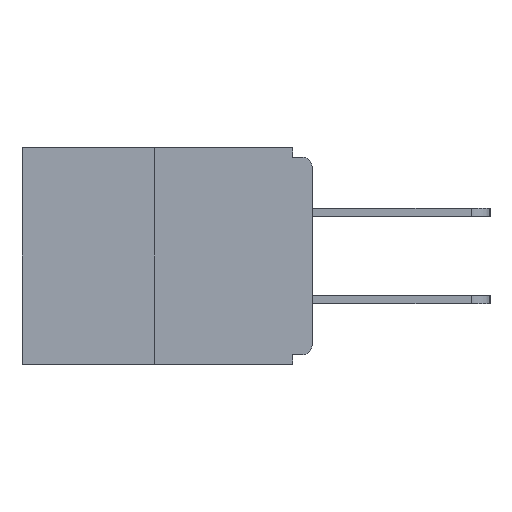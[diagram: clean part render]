
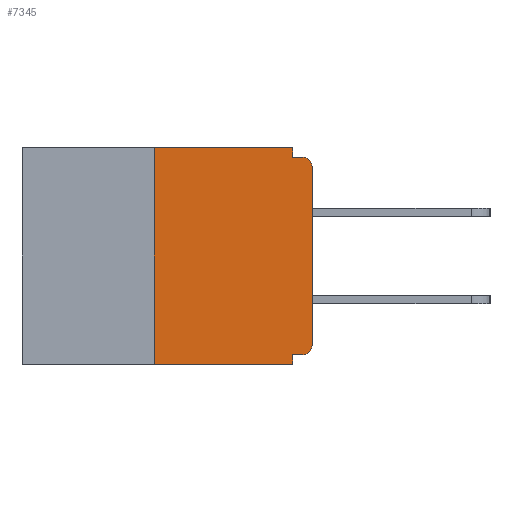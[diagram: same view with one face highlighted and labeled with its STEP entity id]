
A CAD part, left-side view. The second image highlights one B-rep face of the part: STEP entity #7345.
In plain terms, the highlighted planar face has unit normal (-1, 0, 0).
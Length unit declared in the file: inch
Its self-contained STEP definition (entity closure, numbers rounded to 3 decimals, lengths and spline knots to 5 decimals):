
#115 = CARTESIAN_POINT ( 'NONE',  ( 0., 0.015, -0.313 ) ) ;
#485 = EDGE_CURVE ( 'NONE', #3278, #4125, #10283, .T. ) ;
#529 = LINE ( 'NONE', #5410, #9290 ) ;
#544 = CARTESIAN_POINT ( 'NONE',  ( 0., 0.031, -0.328 ) ) ;
#545 = ORIENTED_EDGE ( 'NONE', *, *, #9384, .T. ) ;
#807 = ORIENTED_EDGE ( 'NONE', *, *, #485, .T. ) ;
#889 = EDGE_CURVE ( 'NONE', #6233, #6320, #529, .T. ) ;
#1041 = DIRECTION ( 'NONE',  ( -1., 0., 0. ) ) ;
#1102 = EDGE_CURVE ( 'NONE', #6320, #8349, #2236, .T. ) ;
#1229 = CARTESIAN_POINT ( 'NONE',  ( 0., 0.25, 0. ) ) ;
#1244 = EDGE_CURVE ( 'NONE', #6233, #3278, #9673, .T. ) ;
#1288 = CARTESIAN_POINT ( 'NONE',  ( 0., 0.015, -0.03 ) ) ;
#1404 = VERTEX_POINT ( 'NONE', #2201 ) ;
#1452 = VECTOR ( 'NONE', #3932, 39.37008 ) ;
#2037 = LINE ( 'NONE', #1229, #6083 ) ;
#2065 = VERTEX_POINT ( 'NONE', #5944 ) ;
#2121 = EDGE_LOOP ( 'NONE', ( #9521, #6067, #545, #6357, #8438, #2756, #807, #8352, #10331, #3234 ) ) ;
#2174 = CARTESIAN_POINT ( 'NONE',  ( 0., 0.031, -0.343 ) ) ;
#2178 = VECTOR ( 'NONE', #4045, 39.37008 ) ;
#2180 = LINE ( 'NONE', #8545, #1452 ) ;
#2201 = CARTESIAN_POINT ( 'NONE',  ( 0., 0.031, -0.015 ) ) ;
#2236 = LINE ( 'NONE', #8048, #8984 ) ;
#2301 = VERTEX_POINT ( 'NONE', #6376 ) ;
#2647 = DIRECTION ( 'NONE',  ( 0., -1., 0. ) ) ;
#2756 = ORIENTED_EDGE ( 'NONE', *, *, #1244, .T. ) ;
#3102 = EDGE_CURVE ( 'NONE', #2301, #1404, #2180, .T. ) ;
#3133 = EDGE_CURVE ( 'NONE', #2065, #9595, #2037, .T. ) ;
#3198 = CARTESIAN_POINT ( 'NONE',  ( 0., 0.015, -0.015 ) ) ;
#3234 = ORIENTED_EDGE ( 'NONE', *, *, #3102, .F. ) ;
#3278 = VERTEX_POINT ( 'NONE', #11627 ) ;
#3558 = AXIS2_PLACEMENT_3D ( 'NONE', #6275, #5418, #6326 ) ;
#3870 = DIRECTION ( 'NONE',  ( 0., 0., 1. ) ) ;
#3932 = DIRECTION ( 'NONE',  ( 0., 0., -1. ) ) ;
#3973 = EDGE_CURVE ( 'NONE', #1404, #11168, #7653, .T. ) ;
#4045 = DIRECTION ( 'NONE',  ( 0., -1., 0. ) ) ;
#4125 = VERTEX_POINT ( 'NONE', #6227 ) ;
#4192 = CARTESIAN_POINT ( 'NONE',  ( 0., 0.015, -0.328 ) ) ;
#4301 = DIRECTION ( 'NONE',  ( 0., 0., -1. ) ) ;
#5042 = VECTOR ( 'NONE', #8241, 39.37008 ) ;
#5065 = AXIS2_PLACEMENT_3D ( 'NONE', #115, #1041, #8439 ) ;
#5102 = LINE ( 'NONE', #6280, #9793 ) ;
#5133 = DIRECTION ( 'NONE',  ( 0., 0., -1. ) ) ;
#5410 = CARTESIAN_POINT ( 'NONE',  ( 0., 0., -0.328 ) ) ;
#5418 = DIRECTION ( 'NONE',  ( 1., 0., 0. ) ) ;
#5657 = CARTESIAN_POINT ( 'NONE',  ( 0., 0., -0.015 ) ) ;
#5944 = CARTESIAN_POINT ( 'NONE',  ( 0., 0.25, -0.343 ) ) ;
#6067 = ORIENTED_EDGE ( 'NONE', *, *, #3133, .F. ) ;
#6083 = VECTOR ( 'NONE', #9527, 39.37008 ) ;
#6227 = CARTESIAN_POINT ( 'NONE',  ( 0., 0., -0.03 ) ) ;
#6233 = VERTEX_POINT ( 'NONE', #4192 ) ;
#6275 = CARTESIAN_POINT ( 'NONE',  ( 0., 0.46, 0. ) ) ;
#6280 = CARTESIAN_POINT ( 'NONE',  ( 0., 0.46, -0.343 ) ) ;
#6320 = VERTEX_POINT ( 'NONE', #544 ) ;
#6326 = DIRECTION ( 'NONE',  ( 0., 0., -1. ) ) ;
#6357 = ORIENTED_EDGE ( 'NONE', *, *, #1102, .F. ) ;
#6376 = CARTESIAN_POINT ( 'NONE',  ( 0., 0.031, 0. ) ) ;
#6466 = CARTESIAN_POINT ( 'NONE',  ( 0., 0.25, 0. ) ) ;
#6795 = CARTESIAN_POINT ( 'NONE',  ( 0., 0.46, 0. ) ) ;
#7044 = EDGE_CURVE ( 'NONE', #4125, #11168, #10557, .T. ) ;
#7345 = ADVANCED_FACE ( 'NONE', ( #7578 ), #11805, .F. ) ;
#7578 = FACE_OUTER_BOUND ( 'NONE', #2121, .T. ) ;
#7653 = LINE ( 'NONE', #5657, #5042 ) ;
#8048 = CARTESIAN_POINT ( 'NONE',  ( 0., 0.031, -0.343 ) ) ;
#8241 = DIRECTION ( 'NONE',  ( 0., -1., 0. ) ) ;
#8349 = VERTEX_POINT ( 'NONE', #2174 ) ;
#8352 = ORIENTED_EDGE ( 'NONE', *, *, #7044, .T. ) ;
#8362 = DIRECTION ( 'NONE',  ( 0., 1., 0. ) ) ;
#8438 = ORIENTED_EDGE ( 'NONE', *, *, #889, .F. ) ;
#8439 = DIRECTION ( 'NONE',  ( 0., 0., -1. ) ) ;
#8545 = CARTESIAN_POINT ( 'NONE',  ( 0., 0.031, 0. ) ) ;
#8984 = VECTOR ( 'NONE', #4301, 39.37008 ) ;
#9253 = AXIS2_PLACEMENT_3D ( 'NONE', #1288, #11453, #5133 ) ;
#9290 = VECTOR ( 'NONE', #8362, 39.37008 ) ;
#9369 = CARTESIAN_POINT ( 'NONE',  ( 0., 0., 0. ) ) ;
#9384 = EDGE_CURVE ( 'NONE', #2065, #8349, #5102, .T. ) ;
#9521 = ORIENTED_EDGE ( 'NONE', *, *, #10406, .F. ) ;
#9527 = DIRECTION ( 'NONE',  ( 0., 0., 1. ) ) ;
#9595 = VERTEX_POINT ( 'NONE', #6466 ) ;
#9673 = CIRCLE ( 'NONE', #5065, 0.015 ) ;
#9793 = VECTOR ( 'NONE', #2647, 39.37008 ) ;
#10283 = LINE ( 'NONE', #9369, #11265 ) ;
#10331 = ORIENTED_EDGE ( 'NONE', *, *, #3973, .F. ) ;
#10348 = LINE ( 'NONE', #6795, #2178 ) ;
#10406 = EDGE_CURVE ( 'NONE', #9595, #2301, #10348, .T. ) ;
#10557 = CIRCLE ( 'NONE', #9253, 0.015 ) ;
#11168 = VERTEX_POINT ( 'NONE', #3198 ) ;
#11265 = VECTOR ( 'NONE', #3870, 39.37008 ) ;
#11453 = DIRECTION ( 'NONE',  ( -1., 0., 0. ) ) ;
#11627 = CARTESIAN_POINT ( 'NONE',  ( 0., 0., -0.313 ) ) ;
#11805 = PLANE ( 'NONE',  #3558 ) ;
